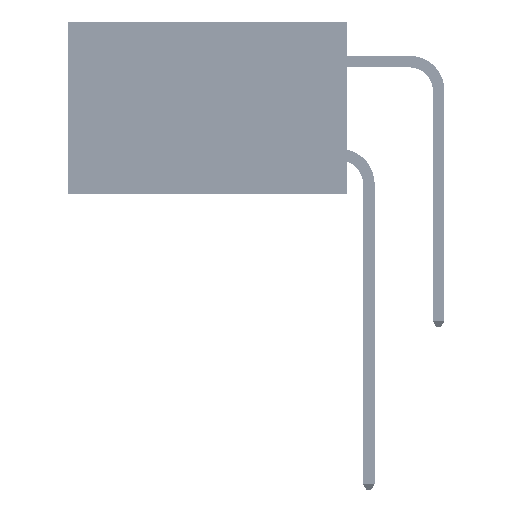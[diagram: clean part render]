
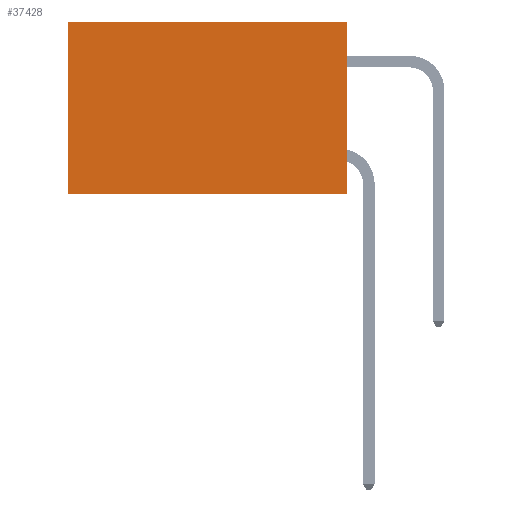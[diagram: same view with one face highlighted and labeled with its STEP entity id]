
A CAD part, left-side view. The second image highlights one B-rep face of the part: STEP entity #37428.
In plain terms, the highlighted planar face has unit normal (-1, 0, 0).
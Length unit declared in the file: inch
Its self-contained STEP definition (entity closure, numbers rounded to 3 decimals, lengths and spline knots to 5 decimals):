
#759 = DIRECTION ( 'NONE',  ( 0., 0., -1. ) ) ;
#3479 = VERTEX_POINT ( 'NONE', #20780 ) ;
#6880 = EDGE_CURVE ( 'NONE', #41142, #39515, #47730, .T. ) ;
#7277 = CARTESIAN_POINT ( 'NONE',  ( 0.2875, 0., -0.37 ) ) ;
#7355 = CARTESIAN_POINT ( 'NONE',  ( 0.2875, 0., 0. ) ) ;
#7824 = CARTESIAN_POINT ( 'NONE',  ( 0.2875, 0., 0. ) ) ;
#11904 = VECTOR ( 'NONE', #24176, 39.37008 ) ;
#16530 = CARTESIAN_POINT ( 'NONE',  ( 0.2875, 0., 0. ) ) ;
#16554 = ORIENTED_EDGE ( 'NONE', *, *, #48163, .F. ) ;
#19103 = LINE ( 'NONE', #43722, #44424 ) ;
#19479 = AXIS2_PLACEMENT_3D ( 'NONE', #16530, #48306, #759 ) ;
#19605 = LINE ( 'NONE', #41508, #30738 ) ;
#19814 = LINE ( 'NONE', #7355, #23513 ) ;
#19903 = DIRECTION ( 'NONE',  ( 0., 1., 0. ) ) ;
#20780 = CARTESIAN_POINT ( 'NONE',  ( 0.2875, 0.6, -0.37 ) ) ;
#22240 = ORIENTED_EDGE ( 'NONE', *, *, #6880, .T. ) ;
#23513 = VECTOR ( 'NONE', #34849, 39.37008 ) ;
#24176 = DIRECTION ( 'NONE',  ( 0., 1., 0. ) ) ;
#27080 = FACE_OUTER_BOUND ( 'NONE', #27725, .T. ) ;
#27725 = EDGE_LOOP ( 'NONE', ( #37811, #16554, #29914, #22240 ) ) ;
#29176 = CARTESIAN_POINT ( 'NONE',  ( 0.2875, 0.6, 0. ) ) ;
#29914 = ORIENTED_EDGE ( 'NONE', *, *, #47332, .F. ) ;
#30738 = VECTOR ( 'NONE', #45514, 39.37008 ) ;
#32481 = CARTESIAN_POINT ( 'NONE',  ( 0.2875, 0., 0. ) ) ;
#33610 = VERTEX_POINT ( 'NONE', #7277 ) ;
#34849 = DIRECTION ( 'NONE',  ( 0., 0., -1. ) ) ;
#37428 = ADVANCED_FACE ( 'NONE', ( #27080 ), #43972, .F. ) ;
#37788 = EDGE_CURVE ( 'NONE', #39515, #3479, #19605, .T. ) ;
#37811 = ORIENTED_EDGE ( 'NONE', *, *, #37788, .T. ) ;
#39515 = VERTEX_POINT ( 'NONE', #29176 ) ;
#41142 = VERTEX_POINT ( 'NONE', #7824 ) ;
#41508 = CARTESIAN_POINT ( 'NONE',  ( 0.2875, 0.6, 0. ) ) ;
#43722 = CARTESIAN_POINT ( 'NONE',  ( 0.2875, 0., -0.37 ) ) ;
#43972 = PLANE ( 'NONE',  #19479 ) ;
#44424 = VECTOR ( 'NONE', #19903, 39.37008 ) ;
#45514 = DIRECTION ( 'NONE',  ( 0., 0., -1. ) ) ;
#47332 = EDGE_CURVE ( 'NONE', #41142, #33610, #19814, .T. ) ;
#47730 = LINE ( 'NONE', #32481, #11904 ) ;
#48163 = EDGE_CURVE ( 'NONE', #33610, #3479, #19103, .T. ) ;
#48306 = DIRECTION ( 'NONE',  ( 1., 0., 0. ) ) ;
